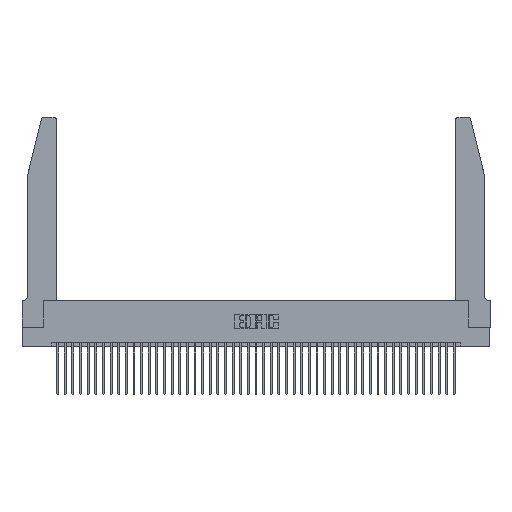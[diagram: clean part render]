
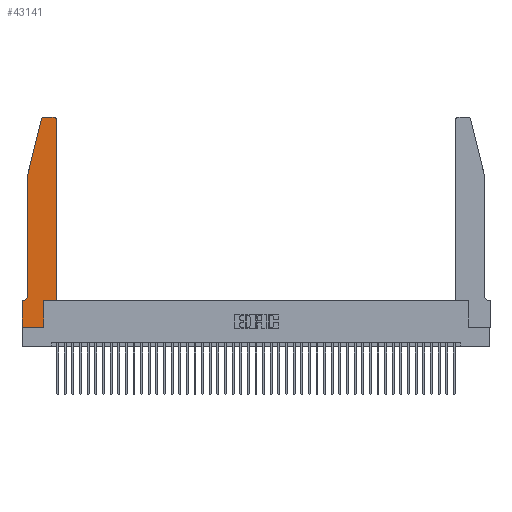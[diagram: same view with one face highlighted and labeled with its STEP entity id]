
A CAD part, top view. The second image highlights one B-rep face of the part: STEP entity #43141.
In plain terms, the highlighted planar face has unit normal (0, 0, 1).
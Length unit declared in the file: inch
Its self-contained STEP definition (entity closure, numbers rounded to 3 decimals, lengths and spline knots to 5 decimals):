
#725 = EDGE_CURVE ( 'NONE', #34424, #33609, #7417, .T. ) ;
#789 = EDGE_CURVE ( 'NONE', #6376, #25557, #4048, .T. ) ;
#946 = ORIENTED_EDGE ( 'NONE', *, *, #17653, .T. ) ;
#1105 = PLANE ( 'NONE',  #36818 ) ;
#1383 = DIRECTION ( 'NONE',  ( 0., 0., 1. ) ) ;
#1596 = VERTEX_POINT ( 'NONE', #7611 ) ;
#1836 = CARTESIAN_POINT ( 'NONE',  ( 0., 0., 0.37 ) ) ;
#2055 = EDGE_CURVE ( 'NONE', #1596, #6376, #17719, .T. ) ;
#2062 = ORIENTED_EDGE ( 'NONE', *, *, #42167, .T. ) ;
#3187 = DIRECTION ( 'NONE',  ( 0., -1., 0. ) ) ;
#3518 = ORIENTED_EDGE ( 'NONE', *, *, #19236, .T. ) ;
#3846 = CARTESIAN_POINT ( 'NONE',  ( 0.2865, 0.35, 0.37 ) ) ;
#4048 = CIRCLE ( 'NONE', #38501, 0.07 ) ;
#4564 = ORIENTED_EDGE ( 'NONE', *, *, #36525, .T. ) ;
#5690 = VECTOR ( 'NONE', #29580, 39.37008 ) ;
#6376 = VERTEX_POINT ( 'NONE', #23962 ) ;
#6957 = CARTESIAN_POINT ( 'NONE',  ( 0.0755, 0.35, 0.37 ) ) ;
#7131 = ORIENTED_EDGE ( 'NONE', *, *, #2055, .T. ) ;
#7274 = VECTOR ( 'NONE', #3187, 39.37008 ) ;
#7417 = LINE ( 'NONE', #40533, #23749 ) ;
#7490 = AXIS2_PLACEMENT_3D ( 'NONE', #36076, #15516, #39491 ) ;
#7611 = CARTESIAN_POINT ( 'NONE',  ( 0.0755, 2., 0.37 ) ) ;
#8162 = CARTESIAN_POINT ( 'NONE',  ( 0.4505, 0.35, 0.37 ) ) ;
#8296 = CARTESIAN_POINT ( 'NONE',  ( 0., 0.35, 0.37 ) ) ;
#8385 = VERTEX_POINT ( 'NONE', #30841 ) ;
#9026 = VECTOR ( 'NONE', #22183, 39.37008 ) ;
#9455 = EDGE_CURVE ( 'NONE', #33609, #10831, #21526, .T. ) ;
#9689 = DIRECTION ( 'NONE',  ( 0., -1., 0. ) ) ;
#9984 = CARTESIAN_POINT ( 'NONE',  ( 0.0055, 0.42, 0.37 ) ) ;
#10297 = LINE ( 'NONE', #30533, #37769 ) ;
#10831 = VERTEX_POINT ( 'NONE', #22072 ) ;
#11835 = DIRECTION ( 'NONE',  ( 1., 0., 0. ) ) ;
#12238 = CARTESIAN_POINT ( 'NONE',  ( 0.0755, 2., 0.37 ) ) ;
#12290 = VECTOR ( 'NONE', #22468, 39.37008 ) ;
#12547 = ORIENTED_EDGE ( 'NONE', *, *, #25486, .T. ) ;
#13360 = DIRECTION ( 'NONE',  ( -1., 0., 0. ) ) ;
#13519 = DIRECTION ( 'NONE',  ( -1., 0., 0. ) ) ;
#14929 = CARTESIAN_POINT ( 'NONE',  ( 0.4205, 2.75, 0.37 ) ) ;
#15065 = LINE ( 'NONE', #12238, #5690 ) ;
#15430 = VERTEX_POINT ( 'NONE', #14929 ) ;
#15516 = DIRECTION ( 'NONE',  ( 0., 0., 1. ) ) ;
#16330 = ORIENTED_EDGE ( 'NONE', *, *, #19992, .T. ) ;
#16558 = EDGE_CURVE ( 'NONE', #20664, #24428, #19168, .T. ) ;
#16597 = CARTESIAN_POINT ( 'NONE',  ( 0., 0.35, 0.37 ) ) ;
#17438 = VECTOR ( 'NONE', #38520, 39.37008 ) ;
#17573 = CARTESIAN_POINT ( 'NONE',  ( 0.4505, 0.35, 0.37 ) ) ;
#17653 = EDGE_CURVE ( 'NONE', #15430, #19504, #10297, .T. ) ;
#17719 = LINE ( 'NONE', #41164, #7274 ) ;
#19144 = CARTESIAN_POINT ( 'NONE',  ( 0.0055, 0.35, 0.37 ) ) ;
#19168 = LINE ( 'NONE', #17573, #20259 ) ;
#19236 = EDGE_CURVE ( 'NONE', #24428, #8385, #35484, .T. ) ;
#19504 = VERTEX_POINT ( 'NONE', #23630 ) ;
#19992 = EDGE_CURVE ( 'NONE', #29325, #1596, #15065, .T. ) ;
#20259 = VECTOR ( 'NONE', #21057, 39.37008 ) ;
#20664 = VERTEX_POINT ( 'NONE', #43139 ) ;
#21057 = DIRECTION ( 'NONE',  ( 1., 0., 0. ) ) ;
#21526 = LINE ( 'NONE', #36084, #12290 ) ;
#21650 = CIRCLE ( 'NONE', #43612, 0.03 ) ;
#22072 = CARTESIAN_POINT ( 'NONE',  ( 0.2865, 0., 0.37 ) ) ;
#22183 = DIRECTION ( 'NONE',  ( 0., 1., 0. ) ) ;
#22428 = CARTESIAN_POINT ( 'NONE',  ( 0.284, 2.72, 0.37 ) ) ;
#22468 = DIRECTION ( 'NONE',  ( 1., 0., 0. ) ) ;
#23630 = CARTESIAN_POINT ( 'NONE',  ( 0.284, 2.75, 0.37 ) ) ;
#23749 = VECTOR ( 'NONE', #9689, 39.37008 ) ;
#23962 = CARTESIAN_POINT ( 'NONE',  ( 0.0755, 0.42, 0.37 ) ) ;
#24428 = VERTEX_POINT ( 'NONE', #39837 ) ;
#24926 = EDGE_CURVE ( 'NONE', #8385, #15430, #27056, .T. ) ;
#25486 = EDGE_CURVE ( 'NONE', #19504, #29325, #21650, .T. ) ;
#25557 = VERTEX_POINT ( 'NONE', #19144 ) ;
#25861 = DIRECTION ( 'NONE',  ( 1., 0., 0. ) ) ;
#26518 = VECTOR ( 'NONE', #31034, 39.37008 ) ;
#27056 = CIRCLE ( 'NONE', #7490, 0.03 ) ;
#27731 = ORIENTED_EDGE ( 'NONE', *, *, #9455, .T. ) ;
#27783 = ORIENTED_EDGE ( 'NONE', *, *, #24926, .T. ) ;
#29067 = ORIENTED_EDGE ( 'NONE', *, *, #16558, .T. ) ;
#29325 = VERTEX_POINT ( 'NONE', #41083 ) ;
#29580 = DIRECTION ( 'NONE',  ( -0.239, -0.971, 0. ) ) ;
#30533 = CARTESIAN_POINT ( 'NONE',  ( 0.2605, 2.75, 0.37 ) ) ;
#30841 = CARTESIAN_POINT ( 'NONE',  ( 0.4505, 2.72, 0.37 ) ) ;
#31034 = DIRECTION ( 'NONE',  ( -1., 0., 0. ) ) ;
#32455 = DIRECTION ( 'NONE',  ( 0., 0., 1. ) ) ;
#33113 = EDGE_LOOP ( 'NONE', ( #946, #12547, #16330, #7131, #37611, #2062, #38027, #27731, #4564, #29067, #3518, #27783 ) ) ;
#33609 = VERTEX_POINT ( 'NONE', #1836 ) ;
#34115 = DIRECTION ( 'NONE',  ( 0., 0., -1. ) ) ;
#34424 = VERTEX_POINT ( 'NONE', #16597 ) ;
#34557 = LINE ( 'NONE', #6957, #26518 ) ;
#35484 = LINE ( 'NONE', #8162, #9026 ) ;
#35682 = LINE ( 'NONE', #3846, #17438 ) ;
#36076 = CARTESIAN_POINT ( 'NONE',  ( 0.4205, 2.72, 0.37 ) ) ;
#36084 = CARTESIAN_POINT ( 'NONE',  ( 0., 0., 0.37 ) ) ;
#36525 = EDGE_CURVE ( 'NONE', #10831, #20664, #35682, .T. ) ;
#36567 = FACE_OUTER_BOUND ( 'NONE', #33113, .T. ) ;
#36818 = AXIS2_PLACEMENT_3D ( 'NONE', #8296, #32455, #11835 ) ;
#37611 = ORIENTED_EDGE ( 'NONE', *, *, #789, .T. ) ;
#37769 = VECTOR ( 'NONE', #13360, 39.37008 ) ;
#38027 = ORIENTED_EDGE ( 'NONE', *, *, #725, .T. ) ;
#38501 = AXIS2_PLACEMENT_3D ( 'NONE', #9984, #34115, #13519 ) ;
#38520 = DIRECTION ( 'NONE',  ( 0., 1., 0. ) ) ;
#39491 = DIRECTION ( 'NONE',  ( 1., 0., 0. ) ) ;
#39837 = CARTESIAN_POINT ( 'NONE',  ( 0.4505, 0.35, 0.37 ) ) ;
#40533 = CARTESIAN_POINT ( 'NONE',  ( 0., 0., 0.37 ) ) ;
#41083 = CARTESIAN_POINT ( 'NONE',  ( 0.25487, 2.72718, 0.37 ) ) ;
#41164 = CARTESIAN_POINT ( 'NONE',  ( 0.0755, 2., 0.37 ) ) ;
#42167 = EDGE_CURVE ( 'NONE', #25557, #34424, #34557, .T. ) ;
#43139 = CARTESIAN_POINT ( 'NONE',  ( 0.2865, 0.35, 0.37 ) ) ;
#43141 = ADVANCED_FACE ( 'NONE', ( #36567 ), #1105, .T. ) ;
#43612 = AXIS2_PLACEMENT_3D ( 'NONE', #22428, #1383, #25861 ) ;
